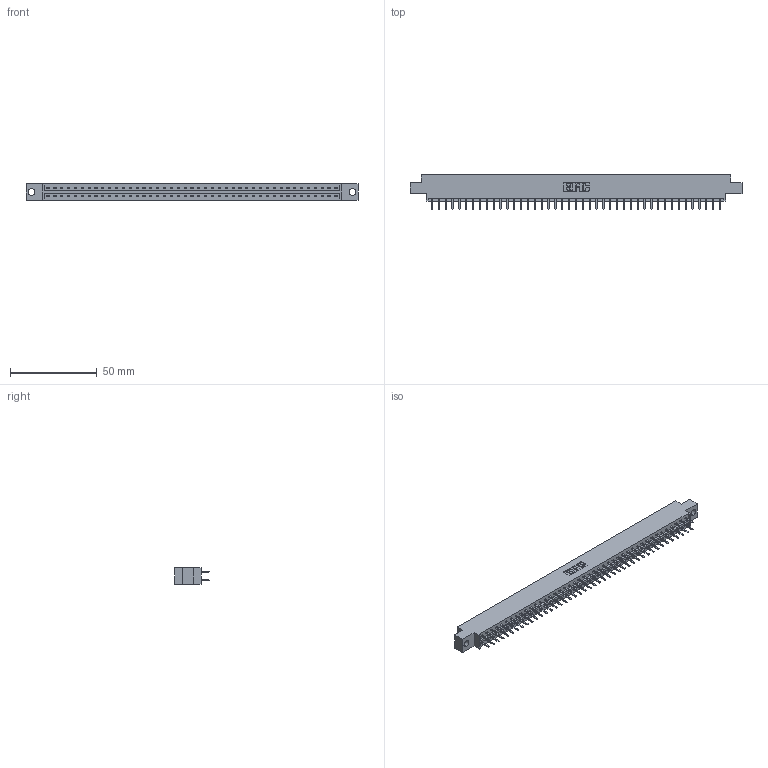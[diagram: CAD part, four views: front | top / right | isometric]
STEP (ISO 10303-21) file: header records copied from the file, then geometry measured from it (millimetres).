
FILE_DESCRIPTION (( 'STEP AP203' ), '1' );
FILE_NAME ('833-086-520-804.STEP', '2020-06-06T02:49:04', ( '' ), ( '' ), 'SwSTEP 2.0', 'SolidWorks 2020', '' );
FILE_SCHEMA (( 'CONFIG_CONTROL_DESIGN' ));
Length unit declared in the file: inch
Products named in the file (3): 345-292-001_345-293-120; 833 Part_Offset - .156 Dia - TH; 833-086-520-804
Assembly tree (87 placements, depth 2):
  833-086-520-804
    833 Part_Offset - .156 Dia - TH
    345-292-001_345-293-120  x86
Bounding box: 191.92 x 20.02 x 9.4 mm (x, y, z)
Volume: 19250.1 mm3; surface area: 22689.2 mm2
Topology: 87 solids, 87 shells, 4934 faces, 14341 edges, 9330 vertices
Faces by surface type: plane 3342, cylinder 1592
Entity records: 27783 total; most frequent: CARTESIAN_POINT 4618, ORIENTED_EDGE 4542, DIRECTION 3931, EDGE_CURVE 2271, LINE 2139, VECTOR 2139, VERTEX_POINT 1510, AXIS2_PLACEMENT_3D 896
